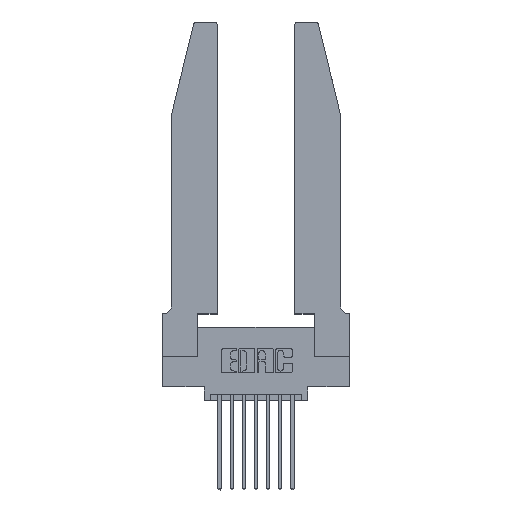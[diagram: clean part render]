
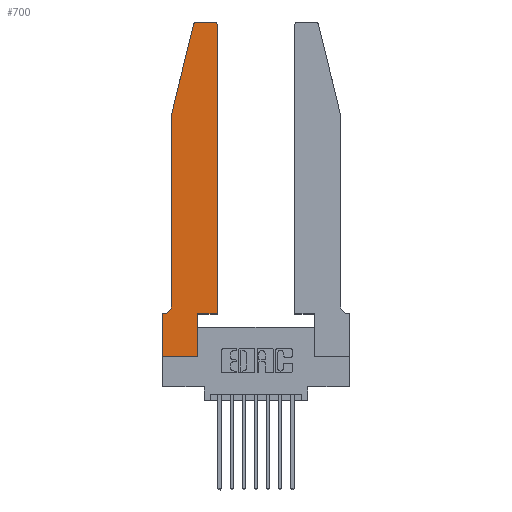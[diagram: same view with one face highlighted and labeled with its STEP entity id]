
A CAD part, top view. The second image highlights one B-rep face of the part: STEP entity #700.
In plain terms, the highlighted planar face has unit normal (0, 0, 1).
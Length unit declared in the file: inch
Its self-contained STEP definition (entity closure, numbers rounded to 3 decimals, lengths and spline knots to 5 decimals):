
#113 = EDGE_CURVE ( 'NONE', #6228, #14068, #6062, .T. ) ;
#248 = CIRCLE ( 'NONE', #11607, 0.03 ) ;
#392 = CARTESIAN_POINT ( 'NONE',  ( 0., 0.35, 0.37 ) ) ;
#445 = EDGE_CURVE ( 'NONE', #1099, #10630, #248, .T. ) ;
#700 = ADVANCED_FACE ( 'NONE', ( #11710 ), #10873, .T. ) ;
#703 = LINE ( 'NONE', #11875, #12596 ) ;
#705 = DIRECTION ( 'NONE',  ( 0., 0., 1. ) ) ;
#738 = CARTESIAN_POINT ( 'NONE',  ( 0., 0., 0.37 ) ) ;
#756 = EDGE_CURVE ( 'NONE', #13338, #10616, #11971, .T. ) ;
#827 = DIRECTION ( 'NONE',  ( 0., 0., 1. ) ) ;
#843 = LINE ( 'NONE', #11275, #9010 ) ;
#896 = DIRECTION ( 'NONE',  ( 0., 1., 0. ) ) ;
#1099 = VERTEX_POINT ( 'NONE', #2130 ) ;
#1179 = CARTESIAN_POINT ( 'NONE',  ( 0.2605, 2.75, 0.37 ) ) ;
#1325 = EDGE_CURVE ( 'NONE', #10616, #12336, #14366, .T. ) ;
#1362 = CARTESIAN_POINT ( 'NONE',  ( 0.0755, 2., 0.37 ) ) ;
#1475 = ORIENTED_EDGE ( 'NONE', *, *, #14868, .T. ) ;
#1561 = DIRECTION ( 'NONE',  ( 1., 0., 0. ) ) ;
#1844 = AXIS2_PLACEMENT_3D ( 'NONE', #9128, #12376, #10514 ) ;
#2003 = VECTOR ( 'NONE', #8427, 39.37008 ) ;
#2062 = AXIS2_PLACEMENT_3D ( 'NONE', #392, #14580, #1561 ) ;
#2116 = CARTESIAN_POINT ( 'NONE',  ( 0.0755, 0.35, 0.37 ) ) ;
#2130 = CARTESIAN_POINT ( 'NONE',  ( 0.4505, 2.72, 0.37 ) ) ;
#2138 = VECTOR ( 'NONE', #13851, 39.37008 ) ;
#2717 = VERTEX_POINT ( 'NONE', #1362 ) ;
#2874 = CARTESIAN_POINT ( 'NONE',  ( 0.284, 2.75, 0.37 ) ) ;
#2990 = ORIENTED_EDGE ( 'NONE', *, *, #5355, .T. ) ;
#3110 = ORIENTED_EDGE ( 'NONE', *, *, #5810, .T. ) ;
#3571 = DIRECTION ( 'NONE',  ( -1., 0., 0. ) ) ;
#3731 = VERTEX_POINT ( 'NONE', #738 ) ;
#4310 = DIRECTION ( 'NONE',  ( 1., 0., 0. ) ) ;
#4378 = DIRECTION ( 'NONE',  ( 1., 0., 0. ) ) ;
#4414 = EDGE_CURVE ( 'NONE', #12336, #3731, #8384, .T. ) ;
#4518 = VERTEX_POINT ( 'NONE', #10180 ) ;
#4616 = DIRECTION ( 'NONE',  ( 0., 1., 0. ) ) ;
#4653 = ORIENTED_EDGE ( 'NONE', *, *, #10195, .T. ) ;
#4761 = CARTESIAN_POINT ( 'NONE',  ( 0., 0.35, 0.37 ) ) ;
#4978 = CARTESIAN_POINT ( 'NONE',  ( 0.4205, 2.75, 0.37 ) ) ;
#5355 = EDGE_CURVE ( 'NONE', #10630, #6228, #5843, .T. ) ;
#5586 = VERTEX_POINT ( 'NONE', #7356 ) ;
#5640 = ORIENTED_EDGE ( 'NONE', *, *, #756, .T. ) ;
#5650 = EDGE_CURVE ( 'NONE', #3731, #5586, #7102, .T. ) ;
#5810 = EDGE_CURVE ( 'NONE', #5586, #4518, #12038, .T. ) ;
#5830 = VECTOR ( 'NONE', #4616, 39.37008 ) ;
#5843 = LINE ( 'NONE', #1179, #8541 ) ;
#6051 = DIRECTION ( 'NONE',  ( -0.239, -0.971, 0. ) ) ;
#6062 = CIRCLE ( 'NONE', #8635, 0.03 ) ;
#6166 = CARTESIAN_POINT ( 'NONE',  ( 0., 0., 0.37 ) ) ;
#6228 = VERTEX_POINT ( 'NONE', #2874 ) ;
#6940 = ORIENTED_EDGE ( 'NONE', *, *, #5650, .T. ) ;
#7102 = LINE ( 'NONE', #10141, #13333 ) ;
#7110 = CARTESIAN_POINT ( 'NONE',  ( 0.0755, 0.42, 0.37 ) ) ;
#7356 = CARTESIAN_POINT ( 'NONE',  ( 0.2865, 0., 0.37 ) ) ;
#7922 = DIRECTION ( 'NONE',  ( 1., 0., 0. ) ) ;
#8384 = LINE ( 'NONE', #6166, #12842 ) ;
#8427 = DIRECTION ( 'NONE',  ( 0., -1., 0. ) ) ;
#8463 = VECTOR ( 'NONE', #7922, 39.37008 ) ;
#8541 = VECTOR ( 'NONE', #3571, 39.37008 ) ;
#8635 = AXIS2_PLACEMENT_3D ( 'NONE', #10055, #827, #4378 ) ;
#8659 = ORIENTED_EDGE ( 'NONE', *, *, #1325, .T. ) ;
#9010 = VECTOR ( 'NONE', #896, 39.37008 ) ;
#9128 = CARTESIAN_POINT ( 'NONE',  ( 0.0055, 0.42, 0.37 ) ) ;
#9946 = CARTESIAN_POINT ( 'NONE',  ( 0.4205, 2.72, 0.37 ) ) ;
#10055 = CARTESIAN_POINT ( 'NONE',  ( 0.284, 2.72, 0.37 ) ) ;
#10124 = EDGE_CURVE ( 'NONE', #2717, #13338, #10369, .T. ) ;
#10141 = CARTESIAN_POINT ( 'NONE',  ( 0., 0., 0.37 ) ) ;
#10180 = CARTESIAN_POINT ( 'NONE',  ( 0.2865, 0.35, 0.37 ) ) ;
#10185 = VERTEX_POINT ( 'NONE', #14172 ) ;
#10195 = EDGE_CURVE ( 'NONE', #14068, #2717, #703, .T. ) ;
#10369 = LINE ( 'NONE', #11781, #2003 ) ;
#10514 = DIRECTION ( 'NONE',  ( -1., 0., 0. ) ) ;
#10616 = VERTEX_POINT ( 'NONE', #14204 ) ;
#10630 = VERTEX_POINT ( 'NONE', #4978 ) ;
#10873 = PLANE ( 'NONE',  #2062 ) ;
#10997 = ORIENTED_EDGE ( 'NONE', *, *, #445, .T. ) ;
#11275 = CARTESIAN_POINT ( 'NONE',  ( 0.4505, 0.35, 0.37 ) ) ;
#11607 = AXIS2_PLACEMENT_3D ( 'NONE', #9946, #705, #12342 ) ;
#11710 = FACE_OUTER_BOUND ( 'NONE', #13509, .T. ) ;
#11781 = CARTESIAN_POINT ( 'NONE',  ( 0.0755, 2., 0.37 ) ) ;
#11875 = CARTESIAN_POINT ( 'NONE',  ( 0.0755, 2., 0.37 ) ) ;
#11971 = CIRCLE ( 'NONE', #1844, 0.07 ) ;
#12038 = LINE ( 'NONE', #14941, #5830 ) ;
#12092 = DIRECTION ( 'NONE',  ( 0., -1., 0. ) ) ;
#12311 = ORIENTED_EDGE ( 'NONE', *, *, #4414, .T. ) ;
#12336 = VERTEX_POINT ( 'NONE', #4761 ) ;
#12342 = DIRECTION ( 'NONE',  ( 1., 0., 0. ) ) ;
#12376 = DIRECTION ( 'NONE',  ( 0., 0., -1. ) ) ;
#12417 = ORIENTED_EDGE ( 'NONE', *, *, #12614, .T. ) ;
#12493 = ORIENTED_EDGE ( 'NONE', *, *, #113, .T. ) ;
#12566 = CARTESIAN_POINT ( 'NONE',  ( 0.4505, 0.35, 0.37 ) ) ;
#12596 = VECTOR ( 'NONE', #6051, 39.37008 ) ;
#12614 = EDGE_CURVE ( 'NONE', #4518, #10185, #12943, .T. ) ;
#12842 = VECTOR ( 'NONE', #12092, 39.37008 ) ;
#12943 = LINE ( 'NONE', #12566, #8463 ) ;
#13195 = CARTESIAN_POINT ( 'NONE',  ( 0.25487, 2.72718, 0.37 ) ) ;
#13333 = VECTOR ( 'NONE', #4310, 39.37008 ) ;
#13338 = VERTEX_POINT ( 'NONE', #7110 ) ;
#13509 = EDGE_LOOP ( 'NONE', ( #2990, #12493, #4653, #14414, #5640, #8659, #12311, #6940, #3110, #12417, #1475, #10997 ) ) ;
#13851 = DIRECTION ( 'NONE',  ( -1., 0., 0. ) ) ;
#14068 = VERTEX_POINT ( 'NONE', #13195 ) ;
#14172 = CARTESIAN_POINT ( 'NONE',  ( 0.4505, 0.35, 0.37 ) ) ;
#14204 = CARTESIAN_POINT ( 'NONE',  ( 0.0055, 0.35, 0.37 ) ) ;
#14366 = LINE ( 'NONE', #2116, #2138 ) ;
#14414 = ORIENTED_EDGE ( 'NONE', *, *, #10124, .T. ) ;
#14580 = DIRECTION ( 'NONE',  ( 0., 0., 1. ) ) ;
#14868 = EDGE_CURVE ( 'NONE', #10185, #1099, #843, .T. ) ;
#14941 = CARTESIAN_POINT ( 'NONE',  ( 0.2865, 0.35, 0.37 ) ) ;
